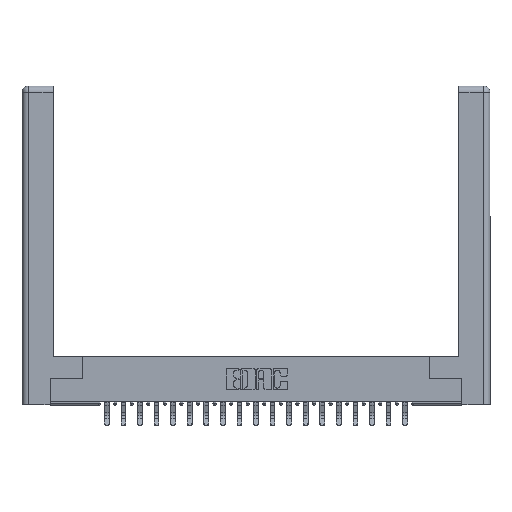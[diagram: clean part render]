
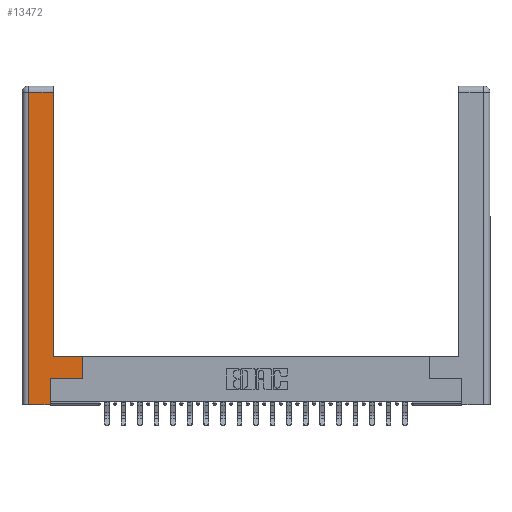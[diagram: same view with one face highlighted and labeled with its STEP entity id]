
A CAD part, top view. The second image highlights one B-rep face of the part: STEP entity #13472.
In plain terms, the highlighted planar face has unit normal (0, 0, 1).
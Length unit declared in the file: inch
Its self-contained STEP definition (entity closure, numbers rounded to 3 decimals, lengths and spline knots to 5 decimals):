
#169 = VERTEX_POINT ( 'NONE', #5780 ) ;
#235 = ORIENTED_EDGE ( 'NONE', *, *, #6160, .T. ) ;
#348 = LINE ( 'NONE', #7470, #14900 ) ;
#537 = DIRECTION ( 'NONE',  ( -1., 0., 0. ) ) ;
#617 = CARTESIAN_POINT ( 'NONE',  ( 0.565, 0.45, 0. ) ) ;
#1194 = VECTOR ( 'NONE', #13421, 39.37008 ) ;
#1282 = CARTESIAN_POINT ( 'NONE',  ( 0.265, 0., 0. ) ) ;
#1618 = VECTOR ( 'NONE', #21475, 39.37008 ) ;
#2099 = CARTESIAN_POINT ( 'NONE',  ( 0.0615, 2.94, 0. ) ) ;
#2368 = AXIS2_PLACEMENT_3D ( 'NONE', #6521, #4645, #537 ) ;
#2925 = CARTESIAN_POINT ( 'NONE',  ( 0.565, 0.45, 0. ) ) ;
#3981 = VECTOR ( 'NONE', #25370, 39.37008 ) ;
#4645 = DIRECTION ( 'NONE',  ( 0., 0., -1. ) ) ;
#4818 = VECTOR ( 'NONE', #10198, 39.37008 ) ;
#4979 = CARTESIAN_POINT ( 'NONE',  ( 0.265, 0.245, 0. ) ) ;
#5292 = VERTEX_POINT ( 'NONE', #16298 ) ;
#5586 = DIRECTION ( 'NONE',  ( -1., 0., 0. ) ) ;
#5779 = CARTESIAN_POINT ( 'NONE',  ( 0.295, 0.45, 0. ) ) ;
#5780 = CARTESIAN_POINT ( 'NONE',  ( 0.265, 0., 0. ) ) ;
#6044 = CARTESIAN_POINT ( 'NONE',  ( 0.565, 0.245, 0. ) ) ;
#6160 = EDGE_CURVE ( 'NONE', #10159, #8123, #8171, .T. ) ;
#6521 = CARTESIAN_POINT ( 'NONE',  ( 0., 0., 0. ) ) ;
#6960 = VERTEX_POINT ( 'NONE', #617 ) ;
#7470 = CARTESIAN_POINT ( 'NONE',  ( 0.265, 0.245, 0. ) ) ;
#7538 = CARTESIAN_POINT ( 'NONE',  ( 0.0615, 0., 0. ) ) ;
#7674 = EDGE_CURVE ( 'NONE', #8123, #7847, #13159, .T. ) ;
#7847 = VERTEX_POINT ( 'NONE', #2099 ) ;
#8123 = VERTEX_POINT ( 'NONE', #13485 ) ;
#8171 = LINE ( 'NONE', #19513, #1194 ) ;
#8442 = ORIENTED_EDGE ( 'NONE', *, *, #22532, .T. ) ;
#9596 = CARTESIAN_POINT ( 'NONE',  ( 0.0615, 0., 0. ) ) ;
#9739 = LINE ( 'NONE', #2925, #22722 ) ;
#9990 = EDGE_CURVE ( 'NONE', #5292, #6960, #9739, .T. ) ;
#10010 = VERTEX_POINT ( 'NONE', #4979 ) ;
#10073 = VERTEX_POINT ( 'NONE', #7538 ) ;
#10159 = VERTEX_POINT ( 'NONE', #5779 ) ;
#10160 = ORIENTED_EDGE ( 'NONE', *, *, #16518, .T. ) ;
#10198 = DIRECTION ( 'NONE',  ( 1., 0., 0. ) ) ;
#11539 = ORIENTED_EDGE ( 'NONE', *, *, #13146, .T. ) ;
#12116 = PLANE ( 'NONE',  #2368 ) ;
#13146 = EDGE_CURVE ( 'NONE', #10010, #5292, #13367, .T. ) ;
#13159 = LINE ( 'NONE', #15683, #21344 ) ;
#13367 = LINE ( 'NONE', #6044, #4818 ) ;
#13421 = DIRECTION ( 'NONE',  ( 0., 1., 0. ) ) ;
#13472 = ADVANCED_FACE ( 'NONE', ( #25074 ), #12116, .F. ) ;
#13485 = CARTESIAN_POINT ( 'NONE',  ( 0.295, 2.94, 0. ) ) ;
#14121 = ORIENTED_EDGE ( 'NONE', *, *, #9990, .T. ) ;
#14611 = ORIENTED_EDGE ( 'NONE', *, *, #7674, .T. ) ;
#14900 = VECTOR ( 'NONE', #23664, 39.37008 ) ;
#15473 = CARTESIAN_POINT ( 'NONE',  ( 0.295, 0.45, 0. ) ) ;
#15683 = CARTESIAN_POINT ( 'NONE',  ( 0.0615, 2.94, 0. ) ) ;
#16298 = CARTESIAN_POINT ( 'NONE',  ( 0.565, 0.245, 0. ) ) ;
#16397 = EDGE_CURVE ( 'NONE', #10073, #169, #25240, .T. ) ;
#16518 = EDGE_CURVE ( 'NONE', #7847, #10073, #20782, .T. ) ;
#17379 = DIRECTION ( 'NONE',  ( 0., 1., 0. ) ) ;
#17499 = DIRECTION ( 'NONE',  ( 0., -1., 0. ) ) ;
#17981 = ORIENTED_EDGE ( 'NONE', *, *, #16397, .T. ) ;
#18401 = EDGE_LOOP ( 'NONE', ( #235, #14611, #10160, #17981, #8442, #11539, #14121, #20566 ) ) ;
#19513 = CARTESIAN_POINT ( 'NONE',  ( 0.295, 3., 0. ) ) ;
#20566 = ORIENTED_EDGE ( 'NONE', *, *, #21888, .T. ) ;
#20782 = LINE ( 'NONE', #9596, #23959 ) ;
#21344 = VECTOR ( 'NONE', #5586, 39.37008 ) ;
#21475 = DIRECTION ( 'NONE',  ( -1., 0., 0. ) ) ;
#21888 = EDGE_CURVE ( 'NONE', #6960, #10159, #22553, .T. ) ;
#22532 = EDGE_CURVE ( 'NONE', #169, #10010, #348, .T. ) ;
#22553 = LINE ( 'NONE', #15473, #1618 ) ;
#22722 = VECTOR ( 'NONE', #17379, 39.37008 ) ;
#23664 = DIRECTION ( 'NONE',  ( 0., 1., 0. ) ) ;
#23959 = VECTOR ( 'NONE', #17499, 39.37008 ) ;
#25074 = FACE_OUTER_BOUND ( 'NONE', #18401, .T. ) ;
#25240 = LINE ( 'NONE', #1282, #3981 ) ;
#25370 = DIRECTION ( 'NONE',  ( 1., 0., 0. ) ) ;
